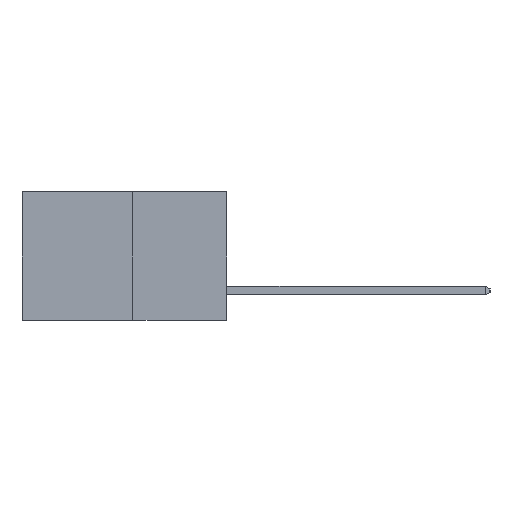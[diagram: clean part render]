
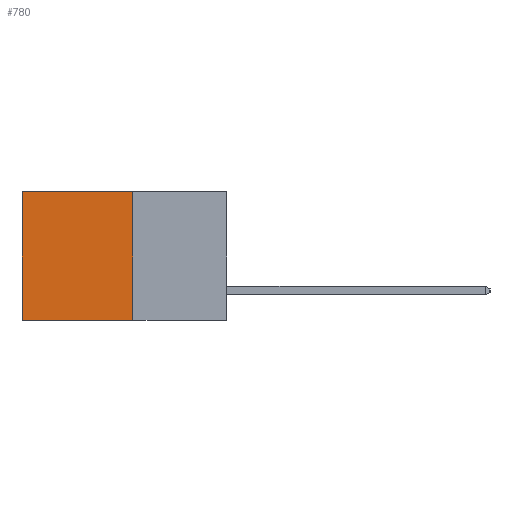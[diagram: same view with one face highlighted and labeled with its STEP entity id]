
A CAD part, left-side view. The second image highlights one B-rep face of the part: STEP entity #780.
In plain terms, the highlighted planar face has unit normal (-1, 0, 0).
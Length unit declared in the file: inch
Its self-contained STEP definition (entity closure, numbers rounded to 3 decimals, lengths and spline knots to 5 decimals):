
#780 = ADVANCED_FACE ( 'NONE', ( #8710 ), #9264, .F. ) ;
#1055 = CARTESIAN_POINT ( 'NONE',  ( 0.277, 0.27, -0.37 ) ) ;
#1781 = VECTOR ( 'NONE', #2352, 39.37008 ) ;
#2184 = DIRECTION ( 'NONE',  ( 0., 1., 0. ) ) ;
#2352 = DIRECTION ( 'NONE',  ( 0., 0., -1. ) ) ;
#2412 = EDGE_LOOP ( 'NONE', ( #12640, #5569, #9574, #11613 ) ) ;
#2785 = CARTESIAN_POINT ( 'NONE',  ( 0.277, 0.27, -0.37 ) ) ;
#3444 = VERTEX_POINT ( 'NONE', #7802 ) ;
#3684 = LINE ( 'NONE', #9265, #4001 ) ;
#4001 = VECTOR ( 'NONE', #2184, 39.37008 ) ;
#4846 = VECTOR ( 'NONE', #10735, 39.37008 ) ;
#5569 = ORIENTED_EDGE ( 'NONE', *, *, #11100, .F. ) ;
#6107 = CARTESIAN_POINT ( 'NONE',  ( 0.277, 0.59, 0. ) ) ;
#6538 = VERTEX_POINT ( 'NONE', #6107 ) ;
#6669 = CARTESIAN_POINT ( 'NONE',  ( 0.277, 0.27, -0.37 ) ) ;
#6685 = CARTESIAN_POINT ( 'NONE',  ( 0.277, 0.27, -0.37 ) ) ;
#7660 = VERTEX_POINT ( 'NONE', #10879 ) ;
#7802 = CARTESIAN_POINT ( 'NONE',  ( 0.277, 0.59, -0.37 ) ) ;
#8710 = FACE_OUTER_BOUND ( 'NONE', #2412, .T. ) ;
#9121 = DIRECTION ( 'NONE',  ( 0., 1., 0. ) ) ;
#9264 = PLANE ( 'NONE',  #12812 ) ;
#9265 = CARTESIAN_POINT ( 'NONE',  ( 0.277, 0.27, 0. ) ) ;
#9435 = CARTESIAN_POINT ( 'NONE',  ( 0.277, 0.59, -0.37 ) ) ;
#9508 = VECTOR ( 'NONE', #9121, 39.37008 ) ;
#9574 = ORIENTED_EDGE ( 'NONE', *, *, #12781, .F. ) ;
#9821 = LINE ( 'NONE', #1055, #9508 ) ;
#10005 = DIRECTION ( 'NONE',  ( 1., 0., 0. ) ) ;
#10223 = LINE ( 'NONE', #6685, #4846 ) ;
#10513 = EDGE_CURVE ( 'NONE', #7660, #6538, #3684, .T. ) ;
#10620 = EDGE_CURVE ( 'NONE', #6538, #3444, #12497, .T. ) ;
#10735 = DIRECTION ( 'NONE',  ( 0., 0., -1. ) ) ;
#10879 = CARTESIAN_POINT ( 'NONE',  ( 0.277, 0.27, 0. ) ) ;
#11100 = EDGE_CURVE ( 'NONE', #12863, #3444, #9821, .T. ) ;
#11613 = ORIENTED_EDGE ( 'NONE', *, *, #10513, .T. ) ;
#12344 = DIRECTION ( 'NONE',  ( 0., 0., -1. ) ) ;
#12497 = LINE ( 'NONE', #9435, #1781 ) ;
#12640 = ORIENTED_EDGE ( 'NONE', *, *, #10620, .T. ) ;
#12781 = EDGE_CURVE ( 'NONE', #7660, #12863, #10223, .T. ) ;
#12812 = AXIS2_PLACEMENT_3D ( 'NONE', #6669, #10005, #12344 ) ;
#12863 = VERTEX_POINT ( 'NONE', #2785 ) ;
